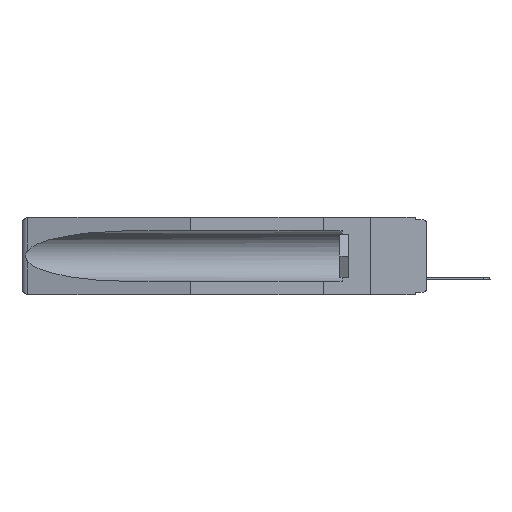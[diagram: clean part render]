
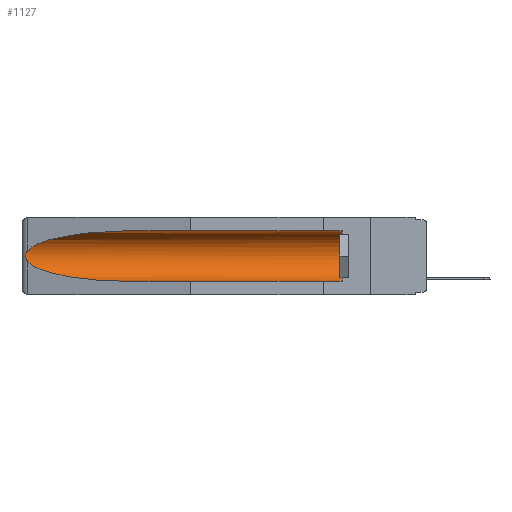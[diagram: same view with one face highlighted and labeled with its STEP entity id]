
A CAD part, left-side view. The second image highlights one B-rep face of the part: STEP entity #1127.
In plain terms, the highlighted cylindrical face has radius 2.857 mm (diameter 5.715 mm), a partial arc.
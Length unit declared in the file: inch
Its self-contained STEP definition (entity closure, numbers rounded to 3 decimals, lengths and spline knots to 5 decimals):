
#829 = CARTESIAN_POINT ( 'NONE',  ( 0.26537, 1.52718, -0.19328 ) ) ;
#1127 = ADVANCED_FACE ( 'NONE', ( #17028 ), #10362, .F. ) ;
#1343 = CARTESIAN_POINT ( 'NONE',  ( 0.26654, 1.53092, -0.15636 ) ) ;
#1415 = ORIENTED_EDGE ( 'NONE', *, *, #10742, .T. ) ;
#1483 = CARTESIAN_POINT ( 'NONE',  ( 0.155, 0.126, -0.1715 ) ) ;
#2564 = CARTESIAN_POINT ( 'NONE',  ( 0.21114, 1.30732, -0.059 ) ) ;
#2953 = CARTESIAN_POINT ( 'NONE',  ( 0.155, 0.126, -0.284 ) ) ;
#3336 = CARTESIAN_POINT ( 'NONE',  ( 0.26597, 1.5296, -0.19026 ) ) ;
#3679 = EDGE_LOOP ( 'NONE', ( #23038, #23368, #12525, #19362, #1415, #17983 ) ) ;
#4259 = VERTEX_POINT ( 'NONE', #14279 ) ;
#5073 = VECTOR ( 'NONE', #14429, 39.37008 ) ;
#5728 = CARTESIAN_POINT ( 'NONE',  ( 0.155, 1.07973, -0.284 ) ) ;
#5813 = CARTESIAN_POINT ( 'NONE',  ( 0.25451, 1.48313, -0.24835 ) ) ;
#7070 = CARTESIAN_POINT ( 'NONE',  ( 0.26655, 1.53094, -0.18657 ) ) ;
#7269 = B_SPLINE_CURVE_WITH_KNOTS ( 'NONE', 3,
 ( #22719, #13098, #1343, #14961, #16297, #10546, #16827, #7070, #3336, #829 ),
 .UNSPECIFIED., .F., .F.,
 ( 4, 2, 2, 2, 4 ),
 ( 0., 0.00029, 0.00058, 0.00087, 0.00117 ),
 .UNSPECIFIED. ) ;
#7349 = EDGE_CURVE ( 'NONE', #22839, #7432, #11456, .T. ) ;
#7432 = VERTEX_POINT ( 'NONE', #16717 ) ;
#7636 = EDGE_CURVE ( 'NONE', #4259, #23085, #13195, .T. ) ;
#8017 = CIRCLE ( 'NONE', #18611, 0.1125 ) ;
#9064 = CARTESIAN_POINT ( 'NONE',  ( 0.155, 1.07973, -0.284 ) ) ;
#9294 = EDGE_CURVE ( 'NONE', #21100, #4259, #7269, .T. ) ;
#9578 = CARTESIAN_POINT ( 'NONE',  ( 0.21114, 1.30732, -0.284 ) ) ;
#9677 = AXIS2_PLACEMENT_3D ( 'NONE', #10338, #10421, #22160 ) ;
#10176 = VERTEX_POINT ( 'NONE', #2953 ) ;
#10218 = CARTESIAN_POINT ( 'NONE',  ( 0.26537, 1.52718, -0.14972 ) ) ;
#10338 = CARTESIAN_POINT ( 'NONE',  ( 0.155, -0.30754, -0.1715 ) ) ;
#10362 = CYLINDRICAL_SURFACE ( 'NONE', #9677, 0.1125 ) ;
#10421 = DIRECTION ( 'NONE',  ( 0., 1., 0. ) ) ;
#10546 = CARTESIAN_POINT ( 'NONE',  ( 0.2675, 1.53308, -0.17534 ) ) ;
#10742 = EDGE_CURVE ( 'NONE', #10176, #22839, #8017, .T. ) ;
#11456 = LINE ( 'NONE', #20449, #5073 ) ;
#12525 = ORIENTED_EDGE ( 'NONE', *, *, #7636, .T. ) ;
#13078 = DIRECTION ( 'NONE',  ( 0., -1., 0. ) ) ;
#13098 = CARTESIAN_POINT ( 'NONE',  ( 0.26597, 1.52961, -0.15275 ) ) ;
#13195 =( BOUNDED_CURVE ( )  B_SPLINE_CURVE ( 3, ( #17450, #5813, #9578, #5728 ),
 .UNSPECIFIED., .F., .F. ) 
 B_SPLINE_CURVE_WITH_KNOTS ( ( 4, 4 ),
 ( 0.1948, 1.5708 ),
 .UNSPECIFIED. ) 
 CURVE ( )  GEOMETRIC_REPRESENTATION_ITEM ( )  RATIONAL_B_SPLINE_CURVE ( ( 1., 0.848, 0.848, 1. ) ) 
 REPRESENTATION_ITEM ( '' )  );
#13782 = CARTESIAN_POINT ( 'NONE',  ( 0.155, -0.30754, -0.284 ) ) ;
#14015 = CARTESIAN_POINT ( 'NONE',  ( 0.155, 1.07973, -0.059 ) ) ;
#14279 = CARTESIAN_POINT ( 'NONE',  ( 0.26537, 1.52718, -0.19328 ) ) ;
#14341 = CARTESIAN_POINT ( 'NONE',  ( 0.25451, 1.48313, -0.09465 ) ) ;
#14429 = DIRECTION ( 'NONE',  ( 0., 1., 0. ) ) ;
#14961 = CARTESIAN_POINT ( 'NONE',  ( 0.2673, 1.5327, -0.16383 ) ) ;
#15508 = DIRECTION ( 'NONE',  ( 0., 1., 0. ) ) ;
#15509 =( BOUNDED_CURVE ( )  B_SPLINE_CURVE ( 3, ( #14015, #2564, #14341, #16275 ),
 .UNSPECIFIED., .F., .F. ) 
 B_SPLINE_CURVE_WITH_KNOTS ( ( 4, 4 ),
 ( 4.71239, 6.08839 ),
 .UNSPECIFIED. ) 
 CURVE ( )  GEOMETRIC_REPRESENTATION_ITEM ( )  RATIONAL_B_SPLINE_CURVE ( ( 1., 0.848, 0.848, 1. ) ) 
 REPRESENTATION_ITEM ( '' )  );
#15732 = EDGE_CURVE ( 'NONE', #7432, #21100, #15509, .T. ) ;
#16275 = CARTESIAN_POINT ( 'NONE',  ( 0.26537, 1.52718, -0.14972 ) ) ;
#16297 = CARTESIAN_POINT ( 'NONE',  ( 0.2675, 1.53308, -0.16763 ) ) ;
#16717 = CARTESIAN_POINT ( 'NONE',  ( 0.155, 1.07973, -0.059 ) ) ;
#16827 = CARTESIAN_POINT ( 'NONE',  ( 0.2673, 1.53269, -0.17917 ) ) ;
#17028 = FACE_OUTER_BOUND ( 'NONE', #3679, .T. ) ;
#17214 = VECTOR ( 'NONE', #15508, 39.37008 ) ;
#17450 = CARTESIAN_POINT ( 'NONE',  ( 0.26537, 1.52718, -0.19328 ) ) ;
#17497 = LINE ( 'NONE', #13782, #17214 ) ;
#17884 = CARTESIAN_POINT ( 'NONE',  ( 0.155, 0.126, -0.059 ) ) ;
#17983 = ORIENTED_EDGE ( 'NONE', *, *, #7349, .T. ) ;
#18611 = AXIS2_PLACEMENT_3D ( 'NONE', #1483, #13078, #22697 ) ;
#19362 = ORIENTED_EDGE ( 'NONE', *, *, #24524, .F. ) ;
#20449 = CARTESIAN_POINT ( 'NONE',  ( 0.155, -0.30754, -0.059 ) ) ;
#21100 = VERTEX_POINT ( 'NONE', #10218 ) ;
#22160 = DIRECTION ( 'NONE',  ( 0., 0., 1. ) ) ;
#22697 = DIRECTION ( 'NONE',  ( 0., 0., 1. ) ) ;
#22719 = CARTESIAN_POINT ( 'NONE',  ( 0.26537, 1.52718, -0.14972 ) ) ;
#22839 = VERTEX_POINT ( 'NONE', #17884 ) ;
#23038 = ORIENTED_EDGE ( 'NONE', *, *, #15732, .T. ) ;
#23085 = VERTEX_POINT ( 'NONE', #9064 ) ;
#23368 = ORIENTED_EDGE ( 'NONE', *, *, #9294, .T. ) ;
#24524 = EDGE_CURVE ( 'NONE', #10176, #23085, #17497, .T. ) ;
